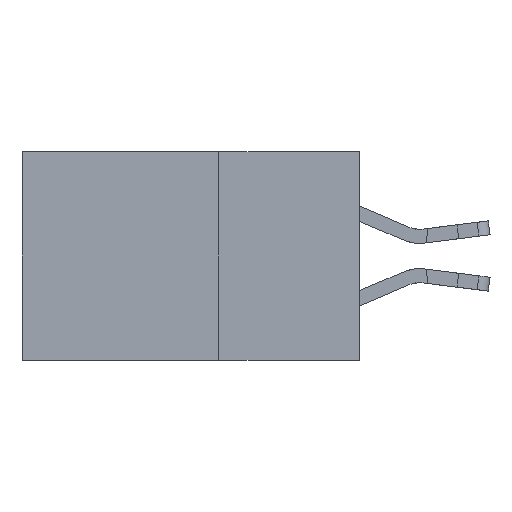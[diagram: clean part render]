
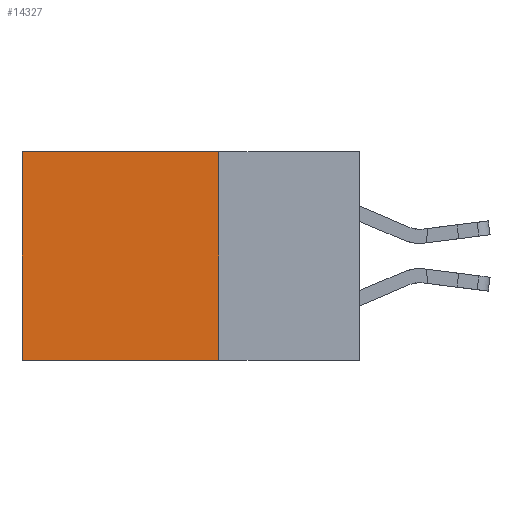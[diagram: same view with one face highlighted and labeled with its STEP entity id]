
A CAD part, left-side view. The second image highlights one B-rep face of the part: STEP entity #14327.
In plain terms, the highlighted planar face has unit normal (-1, 0, 0).
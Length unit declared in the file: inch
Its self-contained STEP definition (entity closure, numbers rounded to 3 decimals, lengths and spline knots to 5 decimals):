
#255 = CARTESIAN_POINT ( 'NONE',  ( 0.2875, 0.25, -0.37 ) ) ;
#606 = ORIENTED_EDGE ( 'NONE', *, *, #19480, .T. ) ;
#1560 = EDGE_CURVE ( 'NONE', #23689, #19623, #10323, .T. ) ;
#1795 = ORIENTED_EDGE ( 'NONE', *, *, #20810, .T. ) ;
#1950 = VECTOR ( 'NONE', #20546, 39.37008 ) ;
#2193 = CARTESIAN_POINT ( 'NONE',  ( 0.2875, 0.25, -0.37 ) ) ;
#2429 = EDGE_CURVE ( 'NONE', #19623, #15850, #21714, .T. ) ;
#2494 = VECTOR ( 'NONE', #2673, 39.37008 ) ;
#2673 = DIRECTION ( 'NONE',  ( 0., 1., 0. ) ) ;
#4272 = CARTESIAN_POINT ( 'NONE',  ( 0.2875, 0.6, -0.37 ) ) ;
#5996 = FACE_OUTER_BOUND ( 'NONE', #10300, .T. ) ;
#6313 = DIRECTION ( 'NONE',  ( 0., 1., 0. ) ) ;
#6396 = VECTOR ( 'NONE', #6313, 39.37008 ) ;
#6496 = DIRECTION ( 'NONE',  ( 1., 0., 0. ) ) ;
#7283 = CARTESIAN_POINT ( 'NONE',  ( 0.2875, 0.25, 0. ) ) ;
#8284 = PLANE ( 'NONE',  #14897 ) ;
#8448 = DIRECTION ( 'NONE',  ( 0., 0., -1. ) ) ;
#8884 = DIRECTION ( 'NONE',  ( 0., 0., -1. ) ) ;
#9311 = VERTEX_POINT ( 'NONE', #15898 ) ;
#10300 = EDGE_LOOP ( 'NONE', ( #606, #13381, #23893, #1795 ) ) ;
#10323 = LINE ( 'NONE', #7283, #1950 ) ;
#13381 = ORIENTED_EDGE ( 'NONE', *, *, #2429, .F. ) ;
#13529 = CARTESIAN_POINT ( 'NONE',  ( 0.2875, 0.25, 0. ) ) ;
#14327 = ADVANCED_FACE ( 'NONE', ( #5996 ), #8284, .F. ) ;
#14399 = CARTESIAN_POINT ( 'NONE',  ( 0.2875, 0.6, 0. ) ) ;
#14897 = AXIS2_PLACEMENT_3D ( 'NONE', #21719, #6496, #8448 ) ;
#15673 = LINE ( 'NONE', #13529, #6396 ) ;
#15850 = VERTEX_POINT ( 'NONE', #4272 ) ;
#15898 = CARTESIAN_POINT ( 'NONE',  ( 0.2875, 0.6, 0. ) ) ;
#18916 = VECTOR ( 'NONE', #8884, 39.37008 ) ;
#19480 = EDGE_CURVE ( 'NONE', #9311, #15850, #23409, .T. ) ;
#19623 = VERTEX_POINT ( 'NONE', #2193 ) ;
#20546 = DIRECTION ( 'NONE',  ( 0., 0., -1. ) ) ;
#20810 = EDGE_CURVE ( 'NONE', #23689, #9311, #15673, .T. ) ;
#21714 = LINE ( 'NONE', #255, #2494 ) ;
#21719 = CARTESIAN_POINT ( 'NONE',  ( 0.2875, 0.25, 0. ) ) ;
#21871 = CARTESIAN_POINT ( 'NONE',  ( 0.2875, 0.25, 0. ) ) ;
#23409 = LINE ( 'NONE', #14399, #18916 ) ;
#23689 = VERTEX_POINT ( 'NONE', #21871 ) ;
#23893 = ORIENTED_EDGE ( 'NONE', *, *, #1560, .F. ) ;
